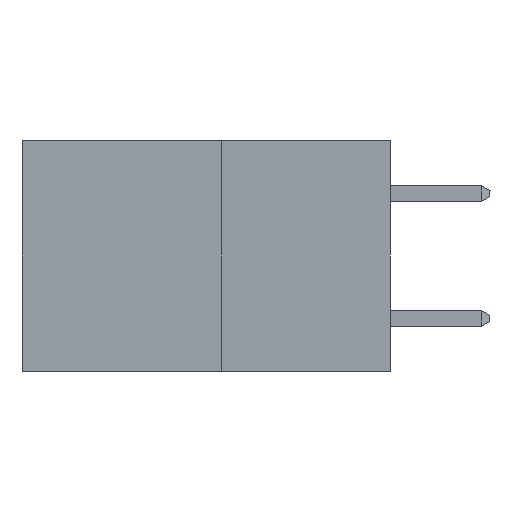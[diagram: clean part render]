
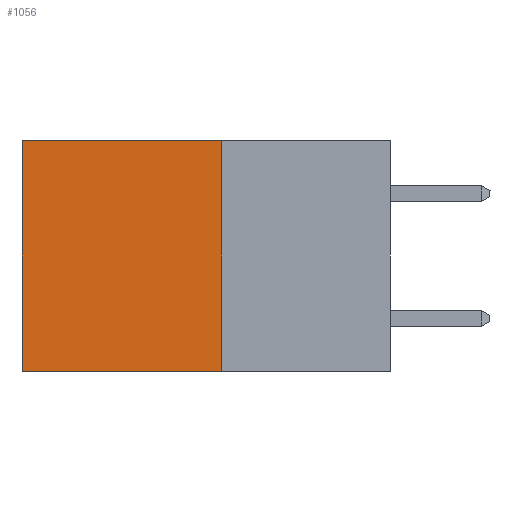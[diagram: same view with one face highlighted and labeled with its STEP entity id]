
A CAD part, left-side view. The second image highlights one B-rep face of the part: STEP entity #1056.
In plain terms, the highlighted planar face has unit normal (-1, 0, 0).
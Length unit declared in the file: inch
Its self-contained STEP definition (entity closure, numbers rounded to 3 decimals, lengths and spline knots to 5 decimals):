
#1056 = ADVANCED_FACE ( 'NONE', ( #6351 ), #8872, .F. ) ;
#1237 = CARTESIAN_POINT ( 'NONE',  ( 0.277, 0.27, -0.37 ) ) ;
#1263 = VECTOR ( 'NONE', #8256, 39.37008 ) ;
#2064 = DIRECTION ( 'NONE',  ( 0., 1., 0. ) ) ;
#2131 = CARTESIAN_POINT ( 'NONE',  ( 0.277, 0.27, -0.37 ) ) ;
#2181 = EDGE_CURVE ( 'NONE', #10956, #6214, #3981, .T. ) ;
#2729 = LINE ( 'NONE', #4782, #10739 ) ;
#2868 = ORIENTED_EDGE ( 'NONE', *, *, #5331, .T. ) ;
#2942 = ORIENTED_EDGE ( 'NONE', *, *, #6696, .F. ) ;
#3098 = ORIENTED_EDGE ( 'NONE', *, *, #10069, .F. ) ;
#3119 = ORIENTED_EDGE ( 'NONE', *, *, #2181, .T. ) ;
#3798 = CARTESIAN_POINT ( 'NONE',  ( 0.277, 0.59, 0. ) ) ;
#3981 = LINE ( 'NONE', #4987, #6057 ) ;
#4051 = CARTESIAN_POINT ( 'NONE',  ( 0.277, 0.27, -0.37 ) ) ;
#4141 = EDGE_LOOP ( 'NONE', ( #2868, #2942, #3098, #3119 ) ) ;
#4649 = DIRECTION ( 'NONE',  ( 1., 0., 0. ) ) ;
#4782 = CARTESIAN_POINT ( 'NONE',  ( 0.277, 0.27, -0.37 ) ) ;
#4886 = VECTOR ( 'NONE', #2064, 39.37008 ) ;
#4987 = CARTESIAN_POINT ( 'NONE',  ( 0.277, 0.27, 0. ) ) ;
#5162 = AXIS2_PLACEMENT_3D ( 'NONE', #1237, #4649, #9354 ) ;
#5331 = EDGE_CURVE ( 'NONE', #6214, #9983, #10182, .T. ) ;
#6057 = VECTOR ( 'NONE', #6365, 39.37008 ) ;
#6214 = VERTEX_POINT ( 'NONE', #3798 ) ;
#6351 = FACE_OUTER_BOUND ( 'NONE', #4141, .T. ) ;
#6365 = DIRECTION ( 'NONE',  ( 0., 1., 0. ) ) ;
#6696 = EDGE_CURVE ( 'NONE', #8489, #9983, #7127, .T. ) ;
#7127 = LINE ( 'NONE', #2131, #4886 ) ;
#8098 = CARTESIAN_POINT ( 'NONE',  ( 0.277, 0.27, 0. ) ) ;
#8150 = DIRECTION ( 'NONE',  ( 0., 0., -1. ) ) ;
#8256 = DIRECTION ( 'NONE',  ( 0., 0., -1. ) ) ;
#8489 = VERTEX_POINT ( 'NONE', #4051 ) ;
#8512 = CARTESIAN_POINT ( 'NONE',  ( 0.277, 0.59, -0.37 ) ) ;
#8872 = PLANE ( 'NONE',  #5162 ) ;
#9354 = DIRECTION ( 'NONE',  ( 0., 0., -1. ) ) ;
#9983 = VERTEX_POINT ( 'NONE', #10472 ) ;
#10069 = EDGE_CURVE ( 'NONE', #10956, #8489, #2729, .T. ) ;
#10182 = LINE ( 'NONE', #8512, #1263 ) ;
#10472 = CARTESIAN_POINT ( 'NONE',  ( 0.277, 0.59, -0.37 ) ) ;
#10739 = VECTOR ( 'NONE', #8150, 39.37008 ) ;
#10956 = VERTEX_POINT ( 'NONE', #8098 ) ;
